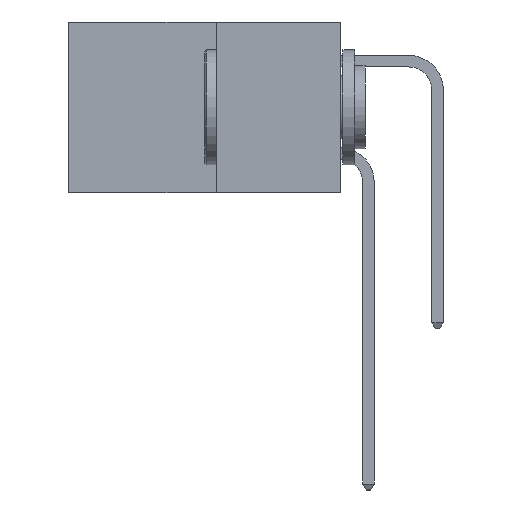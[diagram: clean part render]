
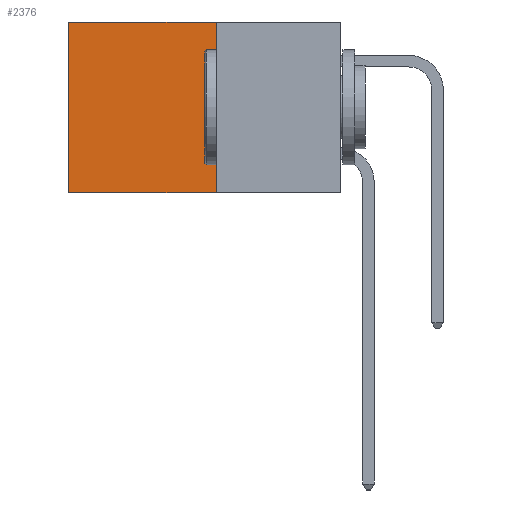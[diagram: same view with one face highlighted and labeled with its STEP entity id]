
A CAD part, left-side view. The second image highlights one B-rep face of the part: STEP entity #2376.
In plain terms, the highlighted planar face has unit normal (-1, 0, 0).
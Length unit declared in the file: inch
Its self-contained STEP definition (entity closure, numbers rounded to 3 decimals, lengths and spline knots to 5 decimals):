
#248 = EDGE_CURVE ( 'NONE', #1889, #3208, #5599, .T. ) ;
#715 = LINE ( 'NONE', #8631, #2764 ) ;
#748 = FACE_OUTER_BOUND ( 'NONE', #5717, .T. ) ;
#825 = CARTESIAN_POINT ( 'NONE',  ( 0.277, 0.59, -0.37 ) ) ;
#1003 = LINE ( 'NONE', #8710, #10076 ) ;
#1437 = VECTOR ( 'NONE', #3327, 39.37008 ) ;
#1889 = VERTEX_POINT ( 'NONE', #1924 ) ;
#1924 = CARTESIAN_POINT ( 'NONE',  ( 0.277, 0.27, -0.37 ) ) ;
#1998 = ORIENTED_EDGE ( 'NONE', *, *, #8666, .T. ) ;
#2037 = CARTESIAN_POINT ( 'NONE',  ( 0.277, 0.59, 0. ) ) ;
#2376 = ADVANCED_FACE ( 'NONE', ( #748 ), #6288, .F. ) ;
#2458 = VERTEX_POINT ( 'NONE', #2037 ) ;
#2764 = VECTOR ( 'NONE', #4264, 39.37008 ) ;
#3208 = VERTEX_POINT ( 'NONE', #825 ) ;
#3275 = VERTEX_POINT ( 'NONE', #11032 ) ;
#3327 = DIRECTION ( 'NONE',  ( 0., 0., -1. ) ) ;
#3560 = VECTOR ( 'NONE', #5330, 39.37008 ) ;
#4264 = DIRECTION ( 'NONE',  ( 0., 1., 0. ) ) ;
#4348 = DIRECTION ( 'NONE',  ( 0., 0., -1. ) ) ;
#5330 = DIRECTION ( 'NONE',  ( 0., 1., 0. ) ) ;
#5599 = LINE ( 'NONE', #8040, #3560 ) ;
#5708 = EDGE_CURVE ( 'NONE', #2458, #3208, #8734, .T. ) ;
#5717 = EDGE_LOOP ( 'NONE', ( #10763, #6237, #6230, #1998 ) ) ;
#6230 = ORIENTED_EDGE ( 'NONE', *, *, #8226, .F. ) ;
#6237 = ORIENTED_EDGE ( 'NONE', *, *, #248, .F. ) ;
#6288 = PLANE ( 'NONE',  #9222 ) ;
#6432 = CARTESIAN_POINT ( 'NONE',  ( 0.277, 0.27, -0.37 ) ) ;
#7137 = DIRECTION ( 'NONE',  ( 1., 0., 0. ) ) ;
#7731 = CARTESIAN_POINT ( 'NONE',  ( 0.277, 0.59, -0.37 ) ) ;
#8040 = CARTESIAN_POINT ( 'NONE',  ( 0.277, 0.27, -0.37 ) ) ;
#8226 = EDGE_CURVE ( 'NONE', #3275, #1889, #1003, .T. ) ;
#8631 = CARTESIAN_POINT ( 'NONE',  ( 0.277, 0.27, 0. ) ) ;
#8666 = EDGE_CURVE ( 'NONE', #3275, #2458, #715, .T. ) ;
#8710 = CARTESIAN_POINT ( 'NONE',  ( 0.277, 0.27, -0.37 ) ) ;
#8734 = LINE ( 'NONE', #7731, #1437 ) ;
#8775 = DIRECTION ( 'NONE',  ( 0., 0., -1. ) ) ;
#9222 = AXIS2_PLACEMENT_3D ( 'NONE', #6432, #7137, #8775 ) ;
#10076 = VECTOR ( 'NONE', #4348, 39.37008 ) ;
#10763 = ORIENTED_EDGE ( 'NONE', *, *, #5708, .T. ) ;
#11032 = CARTESIAN_POINT ( 'NONE',  ( 0.277, 0.27, 0. ) ) ;
